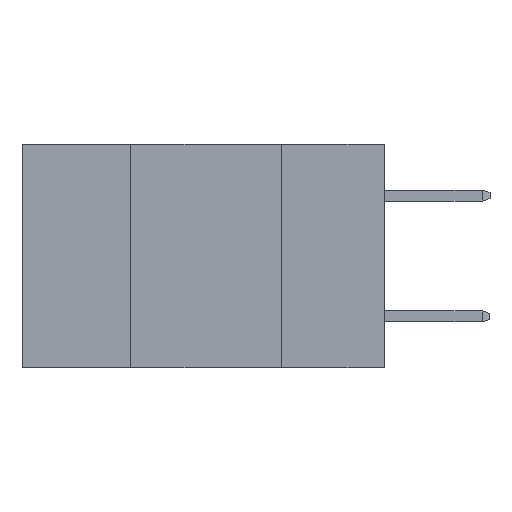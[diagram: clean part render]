
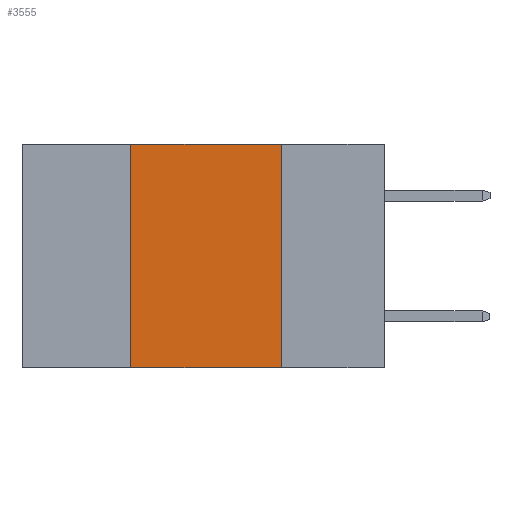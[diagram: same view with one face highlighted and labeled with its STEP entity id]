
A CAD part, left-side view. The second image highlights one B-rep face of the part: STEP entity #3555.
In plain terms, the highlighted planar face has unit normal (-1, 0, 0).
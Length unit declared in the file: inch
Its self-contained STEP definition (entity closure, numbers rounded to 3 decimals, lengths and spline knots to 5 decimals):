
#155 = FACE_OUTER_BOUND ( 'NONE', #7359, .T. ) ;
#848 = EDGE_CURVE ( 'NONE', #4003, #9987, #1734, .T. ) ;
#958 = CARTESIAN_POINT ( 'NONE',  ( 0., 0.42, -0.37 ) ) ;
#978 = CARTESIAN_POINT ( 'NONE',  ( 0., 0.6, 0. ) ) ;
#1164 = PLANE ( 'NONE',  #1551 ) ;
#1551 = AXIS2_PLACEMENT_3D ( 'NONE', #978, #8365, #7885 ) ;
#1695 = DIRECTION ( 'NONE',  ( 0., 0., -1. ) ) ;
#1733 = CARTESIAN_POINT ( 'NONE',  ( 0., 0.6, -0.37 ) ) ;
#1734 = LINE ( 'NONE', #1733, #7667 ) ;
#1744 = ORIENTED_EDGE ( 'NONE', *, *, #6662, .F. ) ;
#1828 = DIRECTION ( 'NONE',  ( 0., -1., 0. ) ) ;
#2346 = VERTEX_POINT ( 'NONE', #3009 ) ;
#2377 = DIRECTION ( 'NONE',  ( 0., -1., 0. ) ) ;
#2607 = ORIENTED_EDGE ( 'NONE', *, *, #6576, .F. ) ;
#3009 = CARTESIAN_POINT ( 'NONE',  ( 0., 0.17, 0. ) ) ;
#3555 = ADVANCED_FACE ( 'NONE', ( #155 ), #1164, .F. ) ;
#4003 = VERTEX_POINT ( 'NONE', #958 ) ;
#4273 = ORIENTED_EDGE ( 'NONE', *, *, #7191, .F. ) ;
#4979 = VECTOR ( 'NONE', #9256, 39.37008 ) ;
#5483 = LINE ( 'NONE', #5715, #4979 ) ;
#5492 = CARTESIAN_POINT ( 'NONE',  ( 0., 0.17, 0. ) ) ;
#5715 = CARTESIAN_POINT ( 'NONE',  ( 0., 0.42, 0. ) ) ;
#6293 = ORIENTED_EDGE ( 'NONE', *, *, #848, .T. ) ;
#6576 = EDGE_CURVE ( 'NONE', #6869, #2346, #9742, .T. ) ;
#6662 = EDGE_CURVE ( 'NONE', #4003, #6869, #5483, .T. ) ;
#6869 = VERTEX_POINT ( 'NONE', #7310 ) ;
#7191 = EDGE_CURVE ( 'NONE', #2346, #9987, #8333, .T. ) ;
#7286 = CARTESIAN_POINT ( 'NONE',  ( 0., 0.17, -0.37 ) ) ;
#7310 = CARTESIAN_POINT ( 'NONE',  ( 0., 0.42, 0. ) ) ;
#7359 = EDGE_LOOP ( 'NONE', ( #4273, #2607, #1744, #6293 ) ) ;
#7667 = VECTOR ( 'NONE', #1828, 39.37008 ) ;
#7764 = VECTOR ( 'NONE', #2377, 39.37008 ) ;
#7885 = DIRECTION ( 'NONE',  ( 0., 0., -1. ) ) ;
#8333 = LINE ( 'NONE', #5492, #8567 ) ;
#8365 = DIRECTION ( 'NONE',  ( 1., 0., 0. ) ) ;
#8567 = VECTOR ( 'NONE', #1695, 39.37008 ) ;
#9256 = DIRECTION ( 'NONE',  ( 0., 0., 1. ) ) ;
#9606 = CARTESIAN_POINT ( 'NONE',  ( 0., 0.6, 0. ) ) ;
#9742 = LINE ( 'NONE', #9606, #7764 ) ;
#9987 = VERTEX_POINT ( 'NONE', #7286 ) ;
